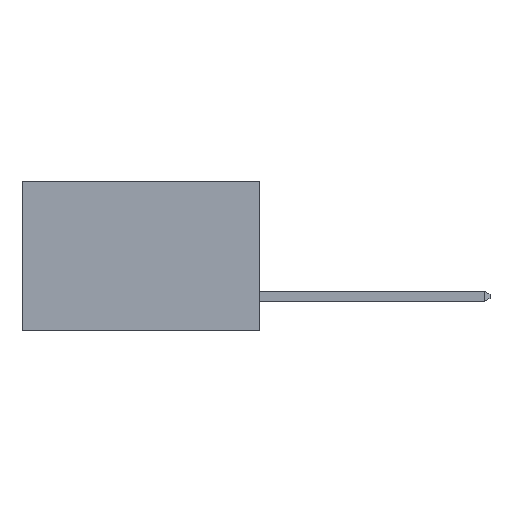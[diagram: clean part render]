
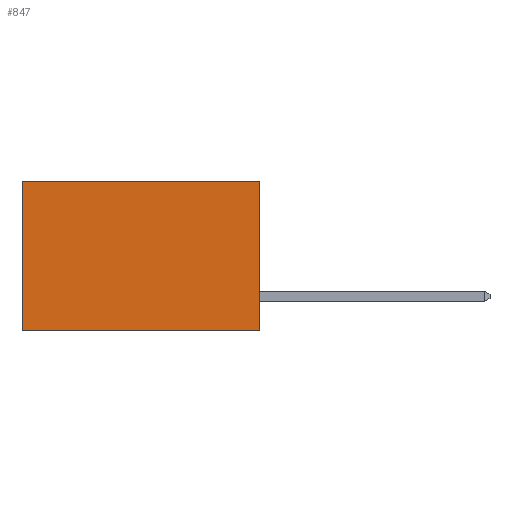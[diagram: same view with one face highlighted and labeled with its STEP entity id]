
A CAD part, left-side view. The second image highlights one B-rep face of the part: STEP entity #847.
In plain terms, the highlighted planar face has unit normal (-1, 0, 0).
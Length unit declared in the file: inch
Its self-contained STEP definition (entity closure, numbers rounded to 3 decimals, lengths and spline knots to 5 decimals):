
#636 = CARTESIAN_POINT ( 'NONE',  ( 0.277, 0., -0.37 ) ) ;
#847 = ADVANCED_FACE ( 'NONE', ( #7383 ), #6276, .F. ) ;
#928 = EDGE_CURVE ( 'NONE', #4132, #3606, #4652, .T. ) ;
#1508 = LINE ( 'NONE', #5323, #6885 ) ;
#1631 = CARTESIAN_POINT ( 'NONE',  ( 0.277, 0., 0. ) ) ;
#1642 = CARTESIAN_POINT ( 'NONE',  ( 0.277, 0.59, -0.37 ) ) ;
#2011 = EDGE_LOOP ( 'NONE', ( #6229, #6277, #6414, #6431 ) ) ;
#2446 = CARTESIAN_POINT ( 'NONE',  ( 0.277, 0., -0.37 ) ) ;
#3265 = EDGE_CURVE ( 'NONE', #7116, #3606, #6541, .T. ) ;
#3330 = VECTOR ( 'NONE', #8618, 39.37008 ) ;
#3421 = EDGE_CURVE ( 'NONE', #7929, #4132, #5205, .T. ) ;
#3606 = VERTEX_POINT ( 'NONE', #5582 ) ;
#3706 = CARTESIAN_POINT ( 'NONE',  ( 0.277, 0.59, 0. ) ) ;
#3801 = DIRECTION ( 'NONE',  ( 0., 0., -1. ) ) ;
#3888 = DIRECTION ( 'NONE',  ( 0., 0., -1. ) ) ;
#4132 = VERTEX_POINT ( 'NONE', #3706 ) ;
#4175 = AXIS2_PLACEMENT_3D ( 'NONE', #2446, #8717, #8563 ) ;
#4652 = LINE ( 'NONE', #1642, #6557 ) ;
#5205 = LINE ( 'NONE', #9032, #3330 ) ;
#5323 = CARTESIAN_POINT ( 'NONE',  ( 0.277, 0., -0.37 ) ) ;
#5582 = CARTESIAN_POINT ( 'NONE',  ( 0.277, 0.59, -0.37 ) ) ;
#6229 = ORIENTED_EDGE ( 'NONE', *, *, #928, .T. ) ;
#6276 = PLANE ( 'NONE',  #4175 ) ;
#6277 = ORIENTED_EDGE ( 'NONE', *, *, #3265, .F. ) ;
#6330 = VECTOR ( 'NONE', #8050, 39.37008 ) ;
#6414 = ORIENTED_EDGE ( 'NONE', *, *, #8701, .F. ) ;
#6431 = ORIENTED_EDGE ( 'NONE', *, *, #3421, .T. ) ;
#6541 = LINE ( 'NONE', #7436, #6330 ) ;
#6557 = VECTOR ( 'NONE', #3801, 39.37008 ) ;
#6885 = VECTOR ( 'NONE', #3888, 39.37008 ) ;
#7116 = VERTEX_POINT ( 'NONE', #636 ) ;
#7383 = FACE_OUTER_BOUND ( 'NONE', #2011, .T. ) ;
#7436 = CARTESIAN_POINT ( 'NONE',  ( 0.277, 0., -0.37 ) ) ;
#7929 = VERTEX_POINT ( 'NONE', #1631 ) ;
#8050 = DIRECTION ( 'NONE',  ( 0., 1., 0. ) ) ;
#8563 = DIRECTION ( 'NONE',  ( 0., 0., -1. ) ) ;
#8618 = DIRECTION ( 'NONE',  ( 0., 1., 0. ) ) ;
#8701 = EDGE_CURVE ( 'NONE', #7929, #7116, #1508, .T. ) ;
#8717 = DIRECTION ( 'NONE',  ( 1., 0., 0. ) ) ;
#9032 = CARTESIAN_POINT ( 'NONE',  ( 0.277, 0., 0. ) ) ;
